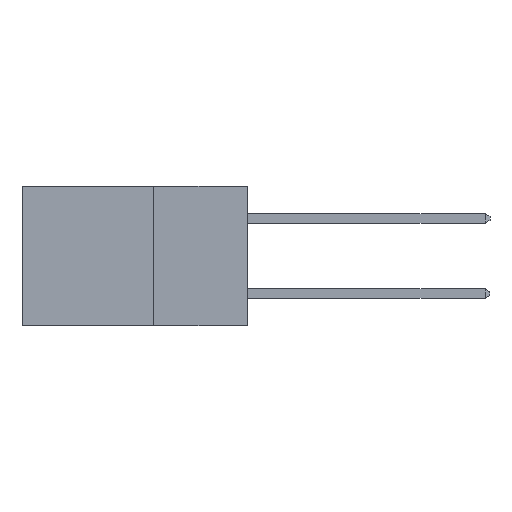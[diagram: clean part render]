
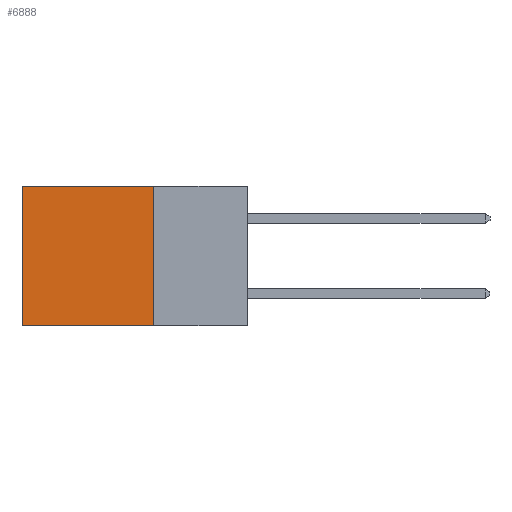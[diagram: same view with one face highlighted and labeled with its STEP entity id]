
A CAD part, left-side view. The second image highlights one B-rep face of the part: STEP entity #6888.
In plain terms, the highlighted planar face has unit normal (-1, 0, 0).
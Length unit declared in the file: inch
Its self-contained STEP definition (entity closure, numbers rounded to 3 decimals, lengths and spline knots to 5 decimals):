
#829 = LINE ( 'NONE', #2201, #1480 ) ;
#969 = EDGE_LOOP ( 'NONE', ( #11450, #5497, #2145, #11222 ) ) ;
#1350 = AXIS2_PLACEMENT_3D ( 'NONE', #12068, #13041, #7121 ) ;
#1480 = VECTOR ( 'NONE', #9388, 39.37008 ) ;
#1502 = EDGE_CURVE ( 'NONE', #11866, #10873, #9226, .T. ) ;
#1720 = DIRECTION ( 'NONE',  ( 0., 1., 0. ) ) ;
#1762 = VERTEX_POINT ( 'NONE', #8361 ) ;
#2145 = ORIENTED_EDGE ( 'NONE', *, *, #6346, .F. ) ;
#2201 = CARTESIAN_POINT ( 'NONE',  ( 0.298, 0.25, 0. ) ) ;
#2908 = EDGE_CURVE ( 'NONE', #10586, #10873, #8095, .T. ) ;
#3492 = FACE_OUTER_BOUND ( 'NONE', #969, .T. ) ;
#5301 = VECTOR ( 'NONE', #12437, 39.37008 ) ;
#5497 = ORIENTED_EDGE ( 'NONE', *, *, #1502, .F. ) ;
#6346 = EDGE_CURVE ( 'NONE', #1762, #11866, #829, .T. ) ;
#6888 = ADVANCED_FACE ( 'NONE', ( #3492 ), #11084, .F. ) ;
#7121 = DIRECTION ( 'NONE',  ( 0., 0., -1. ) ) ;
#7163 = VECTOR ( 'NONE', #9367, 39.37008 ) ;
#7761 = CARTESIAN_POINT ( 'NONE',  ( 0.298, 0.25, -0.37 ) ) ;
#8095 = LINE ( 'NONE', #13044, #5301 ) ;
#8361 = CARTESIAN_POINT ( 'NONE',  ( 0.298, 0.25, 0. ) ) ;
#8627 = CARTESIAN_POINT ( 'NONE',  ( 0.298, 0.25, -0.37 ) ) ;
#9124 = CARTESIAN_POINT ( 'NONE',  ( 0.298, 0.6, -0.37 ) ) ;
#9226 = LINE ( 'NONE', #7761, #11207 ) ;
#9367 = DIRECTION ( 'NONE',  ( 0., 1., 0. ) ) ;
#9388 = DIRECTION ( 'NONE',  ( 0., 0., -1. ) ) ;
#10157 = LINE ( 'NONE', #10366, #7163 ) ;
#10366 = CARTESIAN_POINT ( 'NONE',  ( 0.298, 0.25, 0. ) ) ;
#10586 = VERTEX_POINT ( 'NONE', #11616 ) ;
#10873 = VERTEX_POINT ( 'NONE', #9124 ) ;
#11084 = PLANE ( 'NONE',  #1350 ) ;
#11207 = VECTOR ( 'NONE', #1720, 39.37008 ) ;
#11222 = ORIENTED_EDGE ( 'NONE', *, *, #11728, .T. ) ;
#11450 = ORIENTED_EDGE ( 'NONE', *, *, #2908, .T. ) ;
#11616 = CARTESIAN_POINT ( 'NONE',  ( 0.298, 0.6, 0. ) ) ;
#11728 = EDGE_CURVE ( 'NONE', #1762, #10586, #10157, .T. ) ;
#11866 = VERTEX_POINT ( 'NONE', #8627 ) ;
#12068 = CARTESIAN_POINT ( 'NONE',  ( 0.298, 0.25, 0. ) ) ;
#12437 = DIRECTION ( 'NONE',  ( 0., 0., -1. ) ) ;
#13041 = DIRECTION ( 'NONE',  ( 1., 0., 0. ) ) ;
#13044 = CARTESIAN_POINT ( 'NONE',  ( 0.298, 0.6, 0. ) ) ;
